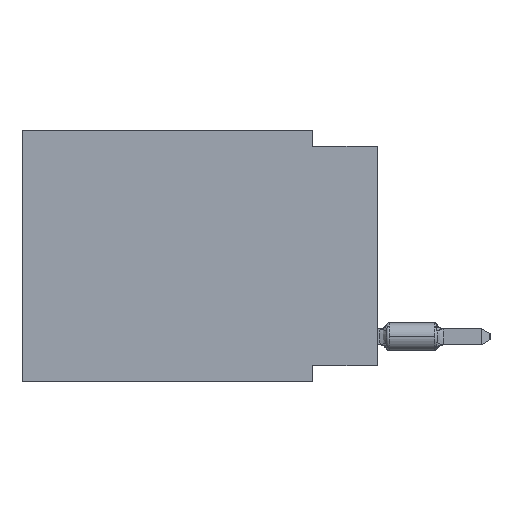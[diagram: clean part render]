
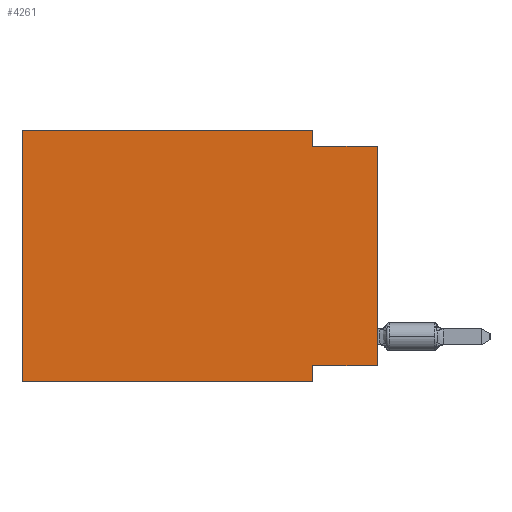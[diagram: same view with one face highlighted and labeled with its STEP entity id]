
A CAD part, left-side view. The second image highlights one B-rep face of the part: STEP entity #4261.
In plain terms, the highlighted planar face has unit normal (-1, 0, 0).
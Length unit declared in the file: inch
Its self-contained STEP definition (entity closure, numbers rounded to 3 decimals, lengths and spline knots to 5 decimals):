
#431 = CARTESIAN_POINT ( 'NONE',  ( 0., 0.1, 0. ) ) ;
#512 = EDGE_CURVE ( 'NONE', #27651, #29799, #4293, .T. ) ;
#786 = CARTESIAN_POINT ( 'NONE',  ( 0., 0.55, 0. ) ) ;
#1379 = LINE ( 'NONE', #21778, #10433 ) ;
#1720 = LINE ( 'NONE', #22280, #20876 ) ;
#1774 = DIRECTION ( 'NONE',  ( 0., 0., -1. ) ) ;
#2954 = LINE ( 'NONE', #431, #3228 ) ;
#3228 = VECTOR ( 'NONE', #10715, 39.37008 ) ;
#3908 = EDGE_CURVE ( 'NONE', #27001, #28456, #14629, .T. ) ;
#4152 = PLANE ( 'NONE',  #8547 ) ;
#4261 = ADVANCED_FACE ( 'NONE', ( #32002 ), #4152, .F. ) ;
#4293 = LINE ( 'NONE', #24880, #28876 ) ;
#5100 = LINE ( 'NONE', #15198, #30183 ) ;
#6450 = EDGE_CURVE ( 'NONE', #15142, #15835, #6948, .T. ) ;
#6596 = ORIENTED_EDGE ( 'NONE', *, *, #23428, .F. ) ;
#6948 = LINE ( 'NONE', #30053, #11199 ) ;
#7619 = CARTESIAN_POINT ( 'NONE',  ( 0., 0.1, -0.365 ) ) ;
#8547 = AXIS2_PLACEMENT_3D ( 'NONE', #8912, #29469, #8572 ) ;
#8572 = DIRECTION ( 'NONE',  ( 0., 0., -1. ) ) ;
#8683 = VERTEX_POINT ( 'NONE', #13761 ) ;
#8724 = CARTESIAN_POINT ( 'NONE',  ( 0., 0.1, -0.39 ) ) ;
#8912 = CARTESIAN_POINT ( 'NONE',  ( 0., 0.55, 0. ) ) ;
#9286 = LINE ( 'NONE', #11805, #17860 ) ;
#9598 = CARTESIAN_POINT ( 'NONE',  ( 0., 0.55, 0. ) ) ;
#10413 = EDGE_CURVE ( 'NONE', #17471, #8683, #2954, .T. ) ;
#10433 = VECTOR ( 'NONE', #24638, 39.37008 ) ;
#10715 = DIRECTION ( 'NONE',  ( 0., 0., -1. ) ) ;
#10751 = ORIENTED_EDGE ( 'NONE', *, *, #6450, .T. ) ;
#11199 = VECTOR ( 'NONE', #19605, 39.37008 ) ;
#11533 = ORIENTED_EDGE ( 'NONE', *, *, #25617, .T. ) ;
#11805 = CARTESIAN_POINT ( 'NONE',  ( 0., 0., -0.025 ) ) ;
#12598 = EDGE_CURVE ( 'NONE', #15142, #27651, #1720, .T. ) ;
#13761 = CARTESIAN_POINT ( 'NONE',  ( 0., 0.1, -0.025 ) ) ;
#14629 = LINE ( 'NONE', #9598, #29892 ) ;
#15142 = VERTEX_POINT ( 'NONE', #32324 ) ;
#15198 = CARTESIAN_POINT ( 'NONE',  ( 0., 0.55, -0.39 ) ) ;
#15532 = DIRECTION ( 'NONE',  ( 0., -1., 0. ) ) ;
#15835 = VERTEX_POINT ( 'NONE', #18750 ) ;
#17214 = DIRECTION ( 'NONE',  ( 0., 1., 0. ) ) ;
#17471 = VERTEX_POINT ( 'NONE', #18550 ) ;
#17860 = VECTOR ( 'NONE', #29529, 39.37008 ) ;
#18407 = ORIENTED_EDGE ( 'NONE', *, *, #512, .F. ) ;
#18550 = CARTESIAN_POINT ( 'NONE',  ( 0., 0.1, 0. ) ) ;
#18750 = CARTESIAN_POINT ( 'NONE',  ( 0., 0., -0.025 ) ) ;
#18806 = EDGE_CURVE ( 'NONE', #8683, #15835, #9286, .T. ) ;
#19605 = DIRECTION ( 'NONE',  ( 0., 0., 1. ) ) ;
#20876 = VECTOR ( 'NONE', #17214, 39.37008 ) ;
#21553 = ORIENTED_EDGE ( 'NONE', *, *, #12598, .F. ) ;
#21778 = CARTESIAN_POINT ( 'NONE',  ( 0., 0.55, 0. ) ) ;
#22280 = CARTESIAN_POINT ( 'NONE',  ( 0., 0., -0.365 ) ) ;
#22847 = ORIENTED_EDGE ( 'NONE', *, *, #3908, .F. ) ;
#23428 = EDGE_CURVE ( 'NONE', #28456, #17471, #1379, .T. ) ;
#23709 = CARTESIAN_POINT ( 'NONE',  ( 0., 0.55, -0.39 ) ) ;
#24638 = DIRECTION ( 'NONE',  ( 0., -1., 0. ) ) ;
#24880 = CARTESIAN_POINT ( 'NONE',  ( 0., 0.1, -0.39 ) ) ;
#25617 = EDGE_CURVE ( 'NONE', #27001, #29799, #5100, .T. ) ;
#27001 = VERTEX_POINT ( 'NONE', #23709 ) ;
#27400 = ORIENTED_EDGE ( 'NONE', *, *, #18806, .F. ) ;
#27651 = VERTEX_POINT ( 'NONE', #7619 ) ;
#28081 = ORIENTED_EDGE ( 'NONE', *, *, #10413, .F. ) ;
#28456 = VERTEX_POINT ( 'NONE', #786 ) ;
#28876 = VECTOR ( 'NONE', #1774, 39.37008 ) ;
#29469 = DIRECTION ( 'NONE',  ( 1., 0., 0. ) ) ;
#29529 = DIRECTION ( 'NONE',  ( 0., -1., 0. ) ) ;
#29799 = VERTEX_POINT ( 'NONE', #8724 ) ;
#29892 = VECTOR ( 'NONE', #30495, 39.37008 ) ;
#30053 = CARTESIAN_POINT ( 'NONE',  ( 0., 0., 0. ) ) ;
#30183 = VECTOR ( 'NONE', #15532, 39.37008 ) ;
#30495 = DIRECTION ( 'NONE',  ( 0., 0., 1. ) ) ;
#32002 = FACE_OUTER_BOUND ( 'NONE', #32669, .T. ) ;
#32324 = CARTESIAN_POINT ( 'NONE',  ( 0., 0., -0.365 ) ) ;
#32669 = EDGE_LOOP ( 'NONE', ( #10751, #27400, #28081, #6596, #22847, #11533, #18407, #21553 ) ) ;
